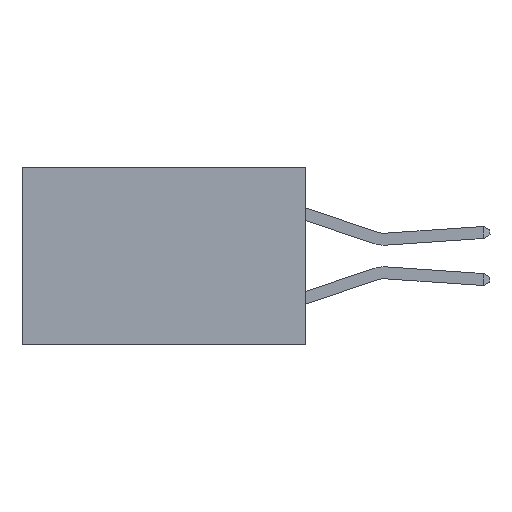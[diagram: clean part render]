
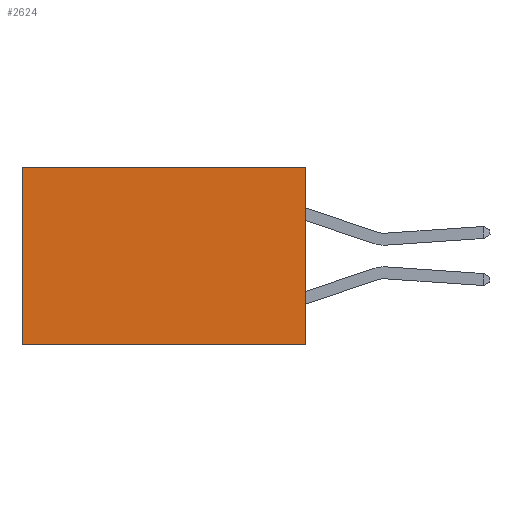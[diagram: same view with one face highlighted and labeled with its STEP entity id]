
A CAD part, left-side view. The second image highlights one B-rep face of the part: STEP entity #2624.
In plain terms, the highlighted planar face has unit normal (-1, 0, 0).
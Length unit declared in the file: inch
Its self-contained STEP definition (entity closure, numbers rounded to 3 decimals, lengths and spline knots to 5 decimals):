
#1131 = ORIENTED_EDGE ( 'NONE', *, *, #11881, .T. ) ;
#1153 = DIRECTION ( 'NONE',  ( 0., 1., 0. ) ) ;
#1485 = CARTESIAN_POINT ( 'NONE',  ( 0.277, 0., -0.37 ) ) ;
#2624 = ADVANCED_FACE ( 'NONE', ( #9527 ), #8048, .F. ) ;
#3005 = DIRECTION ( 'NONE',  ( 0., 0., -1. ) ) ;
#4271 = VECTOR ( 'NONE', #3005, 39.37008 ) ;
#4501 = ORIENTED_EDGE ( 'NONE', *, *, #7172, .F. ) ;
#4779 = EDGE_CURVE ( 'NONE', #5343, #22149, #13991, .T. ) ;
#5096 = VECTOR ( 'NONE', #12556, 39.37008 ) ;
#5343 = VERTEX_POINT ( 'NONE', #5801 ) ;
#5801 = CARTESIAN_POINT ( 'NONE',  ( 0.277, 0.59, 0. ) ) ;
#6094 = EDGE_CURVE ( 'NONE', #7840, #11151, #19223, .T. ) ;
#6624 = LINE ( 'NONE', #1485, #10918 ) ;
#7142 = CARTESIAN_POINT ( 'NONE',  ( 0.277, 0., 0. ) ) ;
#7172 = EDGE_CURVE ( 'NONE', #11151, #22149, #6624, .T. ) ;
#7840 = VERTEX_POINT ( 'NONE', #15644 ) ;
#8048 = PLANE ( 'NONE',  #22299 ) ;
#9527 = FACE_OUTER_BOUND ( 'NONE', #16981, .T. ) ;
#9533 = VECTOR ( 'NONE', #20593, 39.37008 ) ;
#10202 = ORIENTED_EDGE ( 'NONE', *, *, #6094, .F. ) ;
#10918 = VECTOR ( 'NONE', #1153, 39.37008 ) ;
#11151 = VERTEX_POINT ( 'NONE', #12425 ) ;
#11269 = CARTESIAN_POINT ( 'NONE',  ( 0.277, 0.59, -0.37 ) ) ;
#11881 = EDGE_CURVE ( 'NONE', #7840, #5343, #19636, .T. ) ;
#12425 = CARTESIAN_POINT ( 'NONE',  ( 0.277, 0., -0.37 ) ) ;
#12556 = DIRECTION ( 'NONE',  ( 0., 1., 0. ) ) ;
#13991 = LINE ( 'NONE', #11269, #4271 ) ;
#14564 = DIRECTION ( 'NONE',  ( 0., 0., -1. ) ) ;
#15644 = CARTESIAN_POINT ( 'NONE',  ( 0.277, 0., 0. ) ) ;
#16877 = DIRECTION ( 'NONE',  ( 1., 0., 0. ) ) ;
#16981 = EDGE_LOOP ( 'NONE', ( #18916, #4501, #10202, #1131 ) ) ;
#17579 = CARTESIAN_POINT ( 'NONE',  ( 0.277, 0., -0.37 ) ) ;
#18916 = ORIENTED_EDGE ( 'NONE', *, *, #4779, .T. ) ;
#19223 = LINE ( 'NONE', #19902, #9533 ) ;
#19636 = LINE ( 'NONE', #7142, #5096 ) ;
#19902 = CARTESIAN_POINT ( 'NONE',  ( 0.277, 0., -0.37 ) ) ;
#20593 = DIRECTION ( 'NONE',  ( 0., 0., -1. ) ) ;
#22149 = VERTEX_POINT ( 'NONE', #23032 ) ;
#22299 = AXIS2_PLACEMENT_3D ( 'NONE', #17579, #16877, #14564 ) ;
#23032 = CARTESIAN_POINT ( 'NONE',  ( 0.277, 0.59, -0.37 ) ) ;
